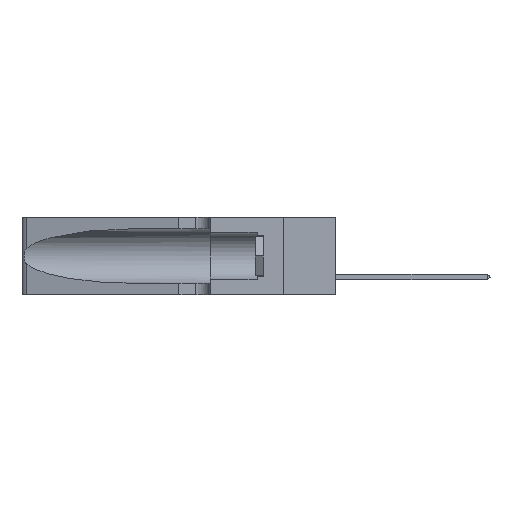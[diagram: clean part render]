
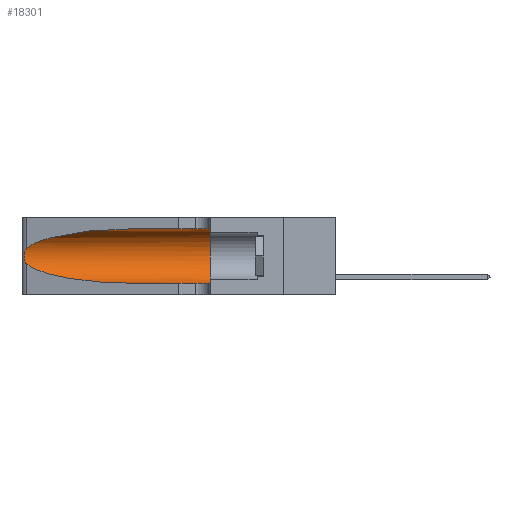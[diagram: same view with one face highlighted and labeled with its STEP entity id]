
A CAD part, left-side view. The second image highlights one B-rep face of the part: STEP entity #18301.
In plain terms, the highlighted cylindrical face has radius 3.308 mm (diameter 6.617 mm), a partial arc.
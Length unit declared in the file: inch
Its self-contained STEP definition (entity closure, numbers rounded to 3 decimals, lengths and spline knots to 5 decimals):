
#130 = B_SPLINE_CURVE_WITH_KNOTS ( 'NONE', 3,
 ( #4887, #20390, #43021, #7070, #28664, #32261, #24704, #29234, #7928, #11364, #40017, #22449, #11207, #40337 ),
 .UNSPECIFIED., .F., .F.,
 ( 4, 2, 2, 2, 2, 2, 4 ),
 ( 0., 0.00027, 0.00053, 0.00107, 0.0016, 0.00187, 0.00214 ),
 .UNSPECIFIED. ) ;
#790 = CARTESIAN_POINT ( 'NONE',  ( 0.2373, 1.15595, 0.28018 ) ) ;
#1138 = CARTESIAN_POINT ( 'NONE',  ( 0.25487, 1.22718, 0.14631 ) ) ;
#1381 = ORIENTED_EDGE ( 'NONE', *, *, #23792, .F. ) ;
#2337 = DIRECTION ( 'NONE',  ( 0., 0., -1. ) ) ;
#4185 = CARTESIAN_POINT ( 'NONE',  ( 0.1305, 1.61858, 0.185 ) ) ;
#4379 = CIRCLE ( 'NONE', #29058, 0.13025 ) ;
#4408 = CARTESIAN_POINT ( 'NONE',  ( 0.25487, 1.22718, 0.22369 ) ) ;
#4887 = CARTESIAN_POINT ( 'NONE',  ( 0.25487, 1.22718, 0.22369 ) ) ;
#5235 = CARTESIAN_POINT ( 'NONE',  ( 0.1305, 0.35, 0.185 ) ) ;
#6321 = CARTESIAN_POINT ( 'NONE',  ( 0.1305, 0.72297, 0.05475 ) ) ;
#6660 = VERTEX_POINT ( 'NONE', #1138 ) ;
#7070 = CARTESIAN_POINT ( 'NONE',  ( 0.25787, 1.23484, 0.2124 ) ) ;
#7928 = CARTESIAN_POINT ( 'NONE',  ( 0.26017, 1.23833, 0.17102 ) ) ;
#8245 = VECTOR ( 'NONE', #12189, 39.37008 ) ;
#9711 = FACE_OUTER_BOUND ( 'NONE', #39371, .T. ) ;
#9949 = EDGE_CURVE ( 'NONE', #6660, #30127, #18716, .T. ) ;
#10790 = EDGE_CURVE ( 'NONE', #30127, #42431, #10828, .T. ) ;
#10828 = LINE ( 'NONE', #32453, #45316 ) ;
#11207 = CARTESIAN_POINT ( 'NONE',  ( 0.25555, 1.22993, 0.14849 ) ) ;
#11364 = CARTESIAN_POINT ( 'NONE',  ( 0.25856, 1.23593, 0.16098 ) ) ;
#11703 = EDGE_CURVE ( 'NONE', #25679, #6660, #130, .T. ) ;
#11825 = EDGE_CURVE ( 'NONE', #31880, #25679, #29786, .T. ) ;
#12086 = LINE ( 'NONE', #22812, #8245 ) ;
#12189 = DIRECTION ( 'NONE',  ( 0., -1., 0. ) ) ;
#15326 = EDGE_CURVE ( 'NONE', #31880, #36960, #12086, .T. ) ;
#16312 = CARTESIAN_POINT ( 'NONE',  ( 0.18966, 0.96281, 0.05475 ) ) ;
#16786 = CARTESIAN_POINT ( 'NONE',  ( 0.25487, 1.22718, 0.14631 ) ) ;
#16904 = ORIENTED_EDGE ( 'NONE', *, *, #11703, .T. ) ;
#18301 = ADVANCED_FACE ( 'NONE', ( #9711 ), #33066, .F. ) ;
#18716 =( BOUNDED_CURVE ( )  B_SPLINE_CURVE ( 3, ( #16786, #34818, #16312, #6321 ),
 .UNSPECIFIED., .F., .T. ) 
 B_SPLINE_CURVE_WITH_KNOTS ( ( 4, 4 ),
 ( 3.44316, 4.71239 ),
 .UNSPECIFIED. ) 
 CURVE ( )  GEOMETRIC_REPRESENTATION_ITEM ( )  RATIONAL_B_SPLINE_CURVE ( ( 1., 0.87, 0.87, 1. ) ) 
 REPRESENTATION_ITEM ( '' )  );
#20144 = AXIS2_PLACEMENT_3D ( 'NONE', #4185, #20163, #2337 ) ;
#20163 = DIRECTION ( 'NONE',  ( 0., -1., 0. ) ) ;
#20390 = CARTESIAN_POINT ( 'NONE',  ( 0.25555, 1.22994, 0.2215 ) ) ;
#21490 = DIRECTION ( 'NONE',  ( 0., -1., 0. ) ) ;
#21757 = CARTESIAN_POINT ( 'NONE',  ( 0.1305, 0.72297, 0.31525 ) ) ;
#21940 = CARTESIAN_POINT ( 'NONE',  ( 0.1305, 0.72297, 0.05475 ) ) ;
#22449 = CARTESIAN_POINT ( 'NONE',  ( 0.25639, 1.23186, 0.15144 ) ) ;
#22812 = CARTESIAN_POINT ( 'NONE',  ( 0.1305, 1.61858, 0.31525 ) ) ;
#23792 = EDGE_CURVE ( 'NONE', #36960, #42431, #4379, .T. ) ;
#24704 = CARTESIAN_POINT ( 'NONE',  ( 0.26075, 1.23896, 0.19203 ) ) ;
#25679 = VERTEX_POINT ( 'NONE', #42011 ) ;
#28664 = CARTESIAN_POINT ( 'NONE',  ( 0.25854, 1.2359, 0.20912 ) ) ;
#29058 = AXIS2_PLACEMENT_3D ( 'NONE', #5235, #30120, #33881 ) ;
#29234 = CARTESIAN_POINT ( 'NONE',  ( 0.26075, 1.23896, 0.178 ) ) ;
#29782 = CARTESIAN_POINT ( 'NONE',  ( 0.18966, 0.96281, 0.31525 ) ) ;
#29786 =( BOUNDED_CURVE ( )  B_SPLINE_CURVE ( 3, ( #32748, #29782, #790, #4408 ),
 .UNSPECIFIED., .F., .F. ) 
 B_SPLINE_CURVE_WITH_KNOTS ( ( 4, 4 ),
 ( 1.5708, 2.84003 ),
 .UNSPECIFIED. ) 
 CURVE ( )  GEOMETRIC_REPRESENTATION_ITEM ( )  RATIONAL_B_SPLINE_CURVE ( ( 1., 0.87, 0.87, 1. ) ) 
 REPRESENTATION_ITEM ( '' )  );
#30120 = DIRECTION ( 'NONE',  ( 0., 1., 0. ) ) ;
#30127 = VERTEX_POINT ( 'NONE', #21940 ) ;
#31880 = VERTEX_POINT ( 'NONE', #21757 ) ;
#32261 = CARTESIAN_POINT ( 'NONE',  ( 0.26018, 1.23835, 0.19895 ) ) ;
#32453 = CARTESIAN_POINT ( 'NONE',  ( 0.1305, 1.61858, 0.05475 ) ) ;
#32748 = CARTESIAN_POINT ( 'NONE',  ( 0.1305, 0.72297, 0.31525 ) ) ;
#33066 = CYLINDRICAL_SURFACE ( 'NONE', #20144, 0.13025 ) ;
#33881 = DIRECTION ( 'NONE',  ( 0., 0., 1. ) ) ;
#34818 = CARTESIAN_POINT ( 'NONE',  ( 0.2373, 1.15595, 0.08982 ) ) ;
#35063 = ORIENTED_EDGE ( 'NONE', *, *, #11825, .T. ) ;
#35780 = ORIENTED_EDGE ( 'NONE', *, *, #9949, .T. ) ;
#36960 = VERTEX_POINT ( 'NONE', #40943 ) ;
#37361 = ORIENTED_EDGE ( 'NONE', *, *, #10790, .T. ) ;
#39371 = EDGE_LOOP ( 'NONE', ( #35063, #16904, #35780, #37361, #1381, #43755 ) ) ;
#40017 = CARTESIAN_POINT ( 'NONE',  ( 0.25789, 1.23486, 0.15765 ) ) ;
#40337 = CARTESIAN_POINT ( 'NONE',  ( 0.25487, 1.22718, 0.14631 ) ) ;
#40943 = CARTESIAN_POINT ( 'NONE',  ( 0.1305, 0.35, 0.31525 ) ) ;
#42011 = CARTESIAN_POINT ( 'NONE',  ( 0.25487, 1.22718, 0.22369 ) ) ;
#42431 = VERTEX_POINT ( 'NONE', #43832 ) ;
#43021 = CARTESIAN_POINT ( 'NONE',  ( 0.25639, 1.23184, 0.21858 ) ) ;
#43755 = ORIENTED_EDGE ( 'NONE', *, *, #15326, .F. ) ;
#43832 = CARTESIAN_POINT ( 'NONE',  ( 0.1305, 0.35, 0.05475 ) ) ;
#45316 = VECTOR ( 'NONE', #21490, 39.37008 ) ;
